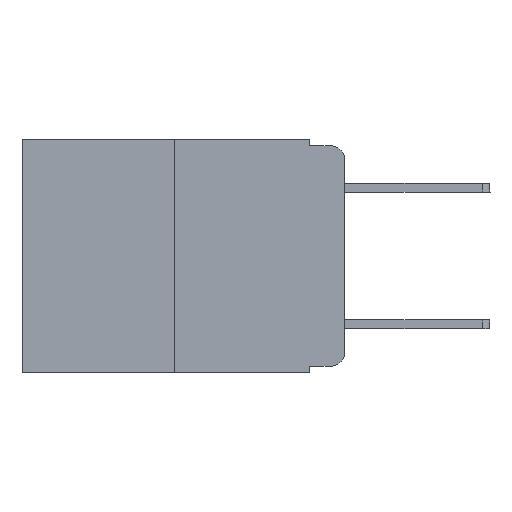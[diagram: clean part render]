
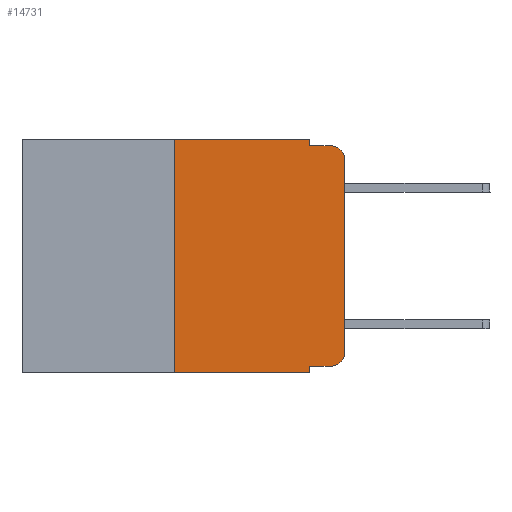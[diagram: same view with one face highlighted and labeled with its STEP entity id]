
A CAD part, left-side view. The second image highlights one B-rep face of the part: STEP entity #14731.
In plain terms, the highlighted planar face has unit normal (-1, 0, 0).
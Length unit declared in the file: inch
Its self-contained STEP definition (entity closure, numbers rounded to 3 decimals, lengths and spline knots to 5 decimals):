
#55 = ORIENTED_EDGE ( 'NONE', *, *, #6769, .F. ) ;
#160 = ORIENTED_EDGE ( 'NONE', *, *, #13699, .T. ) ;
#250 = DIRECTION ( 'NONE',  ( 0., -1., 0. ) ) ;
#301 = EDGE_CURVE ( 'NONE', #17821, #14532, #12242, .T. ) ;
#521 = FACE_OUTER_BOUND ( 'NONE', #14547, .T. ) ;
#621 = CARTESIAN_POINT ( 'NONE',  ( 0., 0.473, 0. ) ) ;
#749 = CARTESIAN_POINT ( 'NONE',  ( 0., 0.051, -0.333 ) ) ;
#794 = DIRECTION ( 'NONE',  ( 0., -1., 0. ) ) ;
#798 = DIRECTION ( 'NONE',  ( 0., 0., -1. ) ) ;
#967 = CARTESIAN_POINT ( 'NONE',  ( 0., 0.051, -0.01 ) ) ;
#1001 = VECTOR ( 'NONE', #14837, 39.37008 ) ;
#1036 = CARTESIAN_POINT ( 'NONE',  ( 0., 0.25, 0. ) ) ;
#1486 = DIRECTION ( 'NONE',  ( -1., 0., 0. ) ) ;
#1603 = VECTOR ( 'NONE', #798, 39.37008 ) ;
#1825 = VECTOR ( 'NONE', #250, 39.37008 ) ;
#1888 = AXIS2_PLACEMENT_3D ( 'NONE', #12377, #17835, #10599 ) ;
#2438 = DIRECTION ( 'NONE',  ( 0., -1., 0. ) ) ;
#2713 = ORIENTED_EDGE ( 'NONE', *, *, #8637, .F. ) ;
#2953 = DIRECTION ( 'NONE',  ( 0., 0., 1. ) ) ;
#3141 = VERTEX_POINT ( 'NONE', #13178 ) ;
#3216 = CARTESIAN_POINT ( 'NONE',  ( 0., 0.473, 0. ) ) ;
#3288 = VERTEX_POINT ( 'NONE', #9651 ) ;
#3954 = LINE ( 'NONE', #14707, #16762 ) ;
#4443 = CARTESIAN_POINT ( 'NONE',  ( 0., 0.25, -0.343 ) ) ;
#4483 = DIRECTION ( 'NONE',  ( 0., 0., -1. ) ) ;
#4506 = ORIENTED_EDGE ( 'NONE', *, *, #14013, .T. ) ;
#4524 = ORIENTED_EDGE ( 'NONE', *, *, #5181, .F. ) ;
#4544 = VECTOR ( 'NONE', #2953, 39.37008 ) ;
#4958 = AXIS2_PLACEMENT_3D ( 'NONE', #3216, #14323, #4483 ) ;
#5181 = EDGE_CURVE ( 'NONE', #17241, #3288, #17725, .T. ) ;
#5622 = CARTESIAN_POINT ( 'NONE',  ( 0., 0.02, -0.333 ) ) ;
#5873 = VERTEX_POINT ( 'NONE', #749 ) ;
#6357 = CARTESIAN_POINT ( 'NONE',  ( 0., 0., -0.03 ) ) ;
#6769 = EDGE_CURVE ( 'NONE', #7027, #3141, #11943, .T. ) ;
#6991 = LINE ( 'NONE', #15303, #4544 ) ;
#7027 = VERTEX_POINT ( 'NONE', #4443 ) ;
#7468 = LINE ( 'NONE', #13323, #1603 ) ;
#7807 = AXIS2_PLACEMENT_3D ( 'NONE', #12479, #1486, #9341 ) ;
#8598 = CARTESIAN_POINT ( 'NONE',  ( 0., 0., -0.313 ) ) ;
#8637 = EDGE_CURVE ( 'NONE', #3288, #14532, #15769, .T. ) ;
#8722 = CARTESIAN_POINT ( 'NONE',  ( 0., 0.051, -0.333 ) ) ;
#8804 = PLANE ( 'NONE',  #4958 ) ;
#8807 = VECTOR ( 'NONE', #13022, 39.37008 ) ;
#8843 = CARTESIAN_POINT ( 'NONE',  ( 0., 0.051, 0. ) ) ;
#9341 = DIRECTION ( 'NONE',  ( 0., 0., -1. ) ) ;
#9651 = CARTESIAN_POINT ( 'NONE',  ( 0., 0.051, -0.01 ) ) ;
#9983 = VECTOR ( 'NONE', #13327, 39.37008 ) ;
#10123 = ORIENTED_EDGE ( 'NONE', *, *, #16515, .F. ) ;
#10206 = EDGE_CURVE ( 'NONE', #17213, #17821, #6991, .T. ) ;
#10599 = DIRECTION ( 'NONE',  ( 0., 0., -1. ) ) ;
#11167 = CARTESIAN_POINT ( 'NONE',  ( 0., 0.051, -0.343 ) ) ;
#11216 = VECTOR ( 'NONE', #794, 39.37008 ) ;
#11283 = LINE ( 'NONE', #8722, #1825 ) ;
#11917 = VERTEX_POINT ( 'NONE', #5622 ) ;
#11943 = LINE ( 'NONE', #1036, #8807 ) ;
#12242 = CIRCLE ( 'NONE', #1888, 0.02 ) ;
#12377 = CARTESIAN_POINT ( 'NONE',  ( 0., 0.02, -0.03 ) ) ;
#12479 = CARTESIAN_POINT ( 'NONE',  ( 0., 0.02, -0.313 ) ) ;
#12645 = ORIENTED_EDGE ( 'NONE', *, *, #10206, .T. ) ;
#13022 = DIRECTION ( 'NONE',  ( 0., 0., 1. ) ) ;
#13178 = CARTESIAN_POINT ( 'NONE',  ( 0., 0.25, 0. ) ) ;
#13323 = CARTESIAN_POINT ( 'NONE',  ( 0., 0.051, 0. ) ) ;
#13327 = DIRECTION ( 'NONE',  ( 0., -1., 0. ) ) ;
#13559 = ORIENTED_EDGE ( 'NONE', *, *, #14713, .T. ) ;
#13699 = EDGE_CURVE ( 'NONE', #11917, #17213, #17594, .T. ) ;
#14013 = EDGE_CURVE ( 'NONE', #7027, #14991, #3954, .T. ) ;
#14299 = ORIENTED_EDGE ( 'NONE', *, *, #301, .T. ) ;
#14323 = DIRECTION ( 'NONE',  ( 1., 0., 0. ) ) ;
#14427 = ORIENTED_EDGE ( 'NONE', *, *, #17785, .F. ) ;
#14532 = VERTEX_POINT ( 'NONE', #16666 ) ;
#14547 = EDGE_LOOP ( 'NONE', ( #12645, #14299, #2713, #4524, #14427, #55, #4506, #10123, #13559, #160 ) ) ;
#14681 = LINE ( 'NONE', #621, #9983 ) ;
#14707 = CARTESIAN_POINT ( 'NONE',  ( 0., 0.473, -0.343 ) ) ;
#14713 = EDGE_CURVE ( 'NONE', #5873, #11917, #11283, .T. ) ;
#14731 = ADVANCED_FACE ( 'NONE', ( #521 ), #8804, .F. ) ;
#14837 = DIRECTION ( 'NONE',  ( 0., 0., -1. ) ) ;
#14991 = VERTEX_POINT ( 'NONE', #11167 ) ;
#15208 = CARTESIAN_POINT ( 'NONE',  ( 0., 0.051, 0. ) ) ;
#15303 = CARTESIAN_POINT ( 'NONE',  ( 0., 0., 0. ) ) ;
#15769 = LINE ( 'NONE', #967, #11216 ) ;
#16515 = EDGE_CURVE ( 'NONE', #5873, #14991, #7468, .T. ) ;
#16666 = CARTESIAN_POINT ( 'NONE',  ( 0., 0.02, -0.01 ) ) ;
#16762 = VECTOR ( 'NONE', #2438, 39.37008 ) ;
#17213 = VERTEX_POINT ( 'NONE', #8598 ) ;
#17241 = VERTEX_POINT ( 'NONE', #8843 ) ;
#17594 = CIRCLE ( 'NONE', #7807, 0.02 ) ;
#17725 = LINE ( 'NONE', #15208, #1001 ) ;
#17785 = EDGE_CURVE ( 'NONE', #3141, #17241, #14681, .T. ) ;
#17821 = VERTEX_POINT ( 'NONE', #6357 ) ;
#17835 = DIRECTION ( 'NONE',  ( -1., 0., 0. ) ) ;
